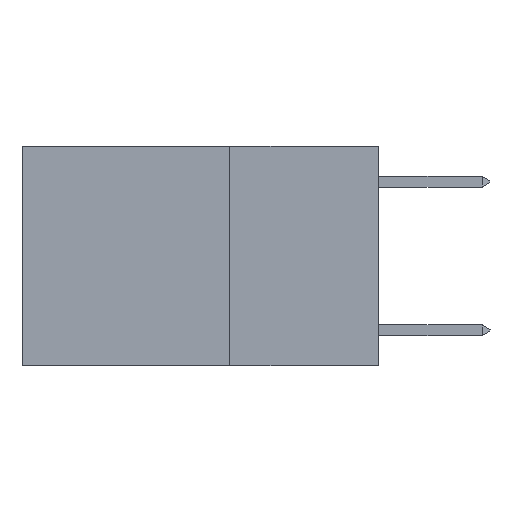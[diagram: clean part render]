
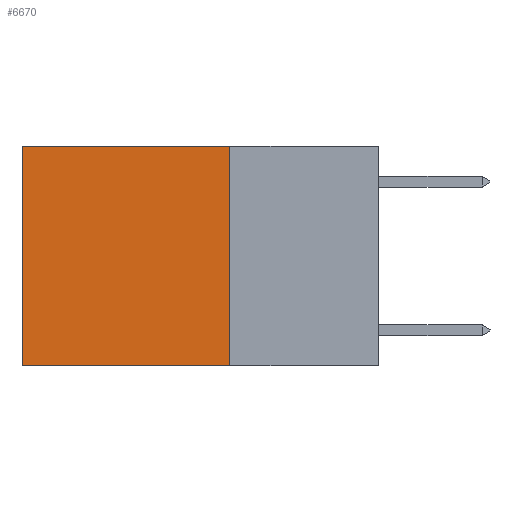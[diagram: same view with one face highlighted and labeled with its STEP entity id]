
A CAD part, left-side view. The second image highlights one B-rep face of the part: STEP entity #6670.
In plain terms, the highlighted planar face has unit normal (-1, 0, 0).
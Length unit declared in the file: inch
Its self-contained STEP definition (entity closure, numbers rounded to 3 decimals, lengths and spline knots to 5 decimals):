
#135 = DIRECTION ( 'NONE',  ( 0., 1., 0. ) ) ;
#417 = EDGE_CURVE ( 'NONE', #1430, #6901, #5282, .T. ) ;
#848 = CARTESIAN_POINT ( 'NONE',  ( 0.2625, 0.25, 0. ) ) ;
#1090 = EDGE_CURVE ( 'NONE', #1430, #4341, #8450, .T. ) ;
#1430 = VERTEX_POINT ( 'NONE', #15376 ) ;
#4163 = CARTESIAN_POINT ( 'NONE',  ( 0.2625, 0.25, -0.37 ) ) ;
#4341 = VERTEX_POINT ( 'NONE', #9434 ) ;
#4610 = ORIENTED_EDGE ( 'NONE', *, *, #4950, .T. ) ;
#4659 = DIRECTION ( 'NONE',  ( 1., 0., 0. ) ) ;
#4877 = DIRECTION ( 'NONE',  ( 0., 0., -1. ) ) ;
#4950 = EDGE_CURVE ( 'NONE', #6901, #12417, #11497, .T. ) ;
#5277 = CARTESIAN_POINT ( 'NONE',  ( 0.2625, 0.6, 0. ) ) ;
#5282 = LINE ( 'NONE', #5895, #14239 ) ;
#5758 = ORIENTED_EDGE ( 'NONE', *, *, #9799, .F. ) ;
#5895 = CARTESIAN_POINT ( 'NONE',  ( 0.2625, 0.25, 0. ) ) ;
#5907 = VECTOR ( 'NONE', #135, 39.37008 ) ;
#6233 = ORIENTED_EDGE ( 'NONE', *, *, #1090, .F. ) ;
#6284 = EDGE_LOOP ( 'NONE', ( #4610, #5758, #6233, #6312 ) ) ;
#6312 = ORIENTED_EDGE ( 'NONE', *, *, #417, .T. ) ;
#6518 = DIRECTION ( 'NONE',  ( 0., 1., 0. ) ) ;
#6670 = ADVANCED_FACE ( 'NONE', ( #12745 ), #10905, .F. ) ;
#6901 = VERTEX_POINT ( 'NONE', #5277 ) ;
#8450 = LINE ( 'NONE', #848, #14379 ) ;
#9434 = CARTESIAN_POINT ( 'NONE',  ( 0.2625, 0.25, -0.37 ) ) ;
#9799 = EDGE_CURVE ( 'NONE', #4341, #12417, #12471, .T. ) ;
#10716 = DIRECTION ( 'NONE',  ( 0., 0., -1. ) ) ;
#10905 = PLANE ( 'NONE',  #14707 ) ;
#11124 = VECTOR ( 'NONE', #10716, 39.37008 ) ;
#11497 = LINE ( 'NONE', #14198, #11124 ) ;
#11881 = CARTESIAN_POINT ( 'NONE',  ( 0.2625, 0.6, -0.37 ) ) ;
#12099 = CARTESIAN_POINT ( 'NONE',  ( 0.2625, 0.25, 0. ) ) ;
#12417 = VERTEX_POINT ( 'NONE', #11881 ) ;
#12471 = LINE ( 'NONE', #4163, #5907 ) ;
#12745 = FACE_OUTER_BOUND ( 'NONE', #6284, .T. ) ;
#13281 = DIRECTION ( 'NONE',  ( 0., 0., -1. ) ) ;
#14198 = CARTESIAN_POINT ( 'NONE',  ( 0.2625, 0.6, 0. ) ) ;
#14239 = VECTOR ( 'NONE', #6518, 39.37008 ) ;
#14379 = VECTOR ( 'NONE', #4877, 39.37008 ) ;
#14707 = AXIS2_PLACEMENT_3D ( 'NONE', #12099, #4659, #13281 ) ;
#15376 = CARTESIAN_POINT ( 'NONE',  ( 0.2625, 0.25, 0. ) ) ;
